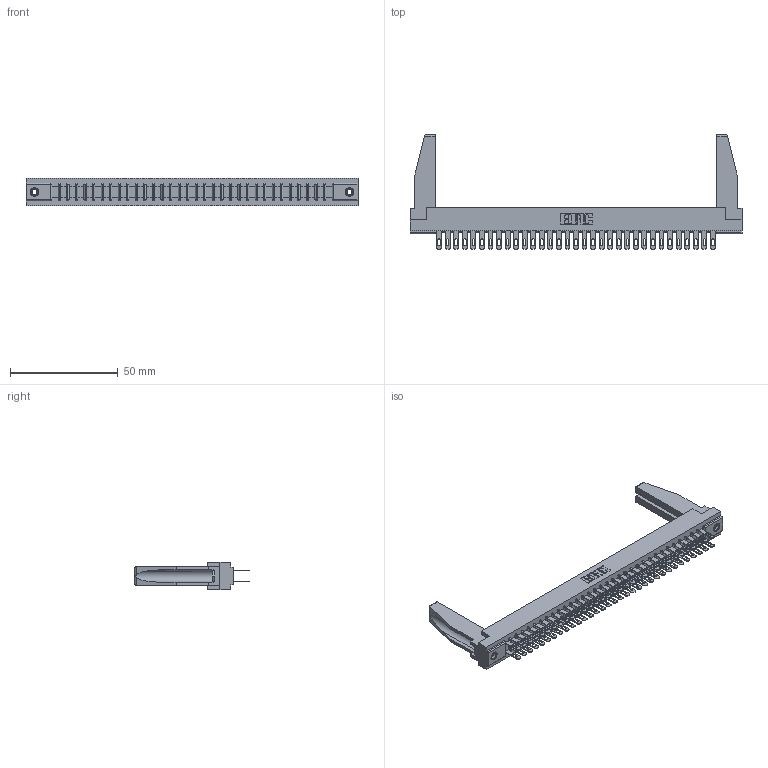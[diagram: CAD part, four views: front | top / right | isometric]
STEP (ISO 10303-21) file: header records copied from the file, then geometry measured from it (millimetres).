
FILE_DESCRIPTION (( 'STEP AP203' ), '1' );
FILE_NAME ('307-066-500-278.STEP', '2019-09-06T17:19:24', ( '' ), ( '' ), 'SwSTEP 2.0', 'SolidWorks 2016', '' );
FILE_SCHEMA (( 'CONFIG_CONTROL_DESIGN' ));
Length unit declared in the file: inch
Products named in the file (5): 307-220-078; 345-250-001_345-250-001-102; 307-290-001_500; 307 Part_.156 Dia Mounting Holes; 307-066-500-278
Assembly tree (71 placements, depth 2):
  307-066-500-278
    307 Part_.156 Dia Mounting Holes
    307-290-001_500  x66
    307-220-078  x2
    345-250-001_345-250-001-102  x2
Bounding box: 153.77 x 52.88 x 12.7 mm (x, y, z)
Volume: 20470.4 mm3; surface area: 24855.9 mm2
Topology: 71 solids, 71 shells, 3318 faces, 9233 edges, 5966 vertices
Faces by surface type: plane 2134, cylinder 1100, sphere 68, cone 12, torus 4
Entity records: 32869 total; most frequent: CARTESIAN_POINT 5387, ORIENTED_EDGE 5296, DIRECTION 5236, EDGE_CURVE 2648, LINE 2030, VECTOR 2030, VERTEX_POINT 1712, AXIS2_PLACEMENT_3D 1603
